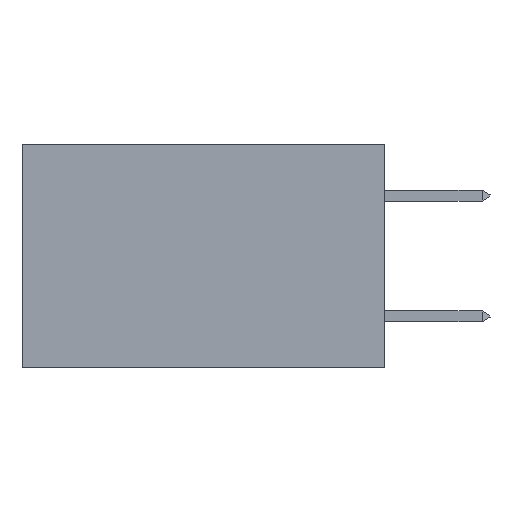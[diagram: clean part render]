
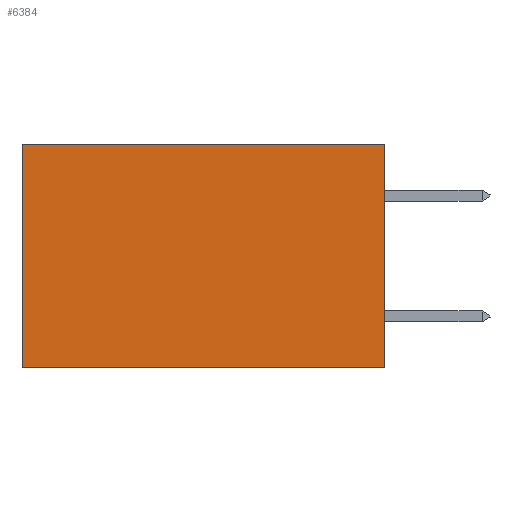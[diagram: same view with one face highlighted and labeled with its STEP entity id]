
A CAD part, left-side view. The second image highlights one B-rep face of the part: STEP entity #6384.
In plain terms, the highlighted planar face has unit normal (-1, 0, 0).
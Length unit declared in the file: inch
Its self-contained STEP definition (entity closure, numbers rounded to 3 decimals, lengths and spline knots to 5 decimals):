
#473 = FACE_OUTER_BOUND ( 'NONE', #5289, .T. ) ;
#729 = VERTEX_POINT ( 'NONE', #10830 ) ;
#1812 = VERTEX_POINT ( 'NONE', #20173 ) ;
#3872 = EDGE_CURVE ( 'NONE', #16620, #5416, #7547, .T. ) ;
#3997 = CARTESIAN_POINT ( 'NONE',  ( 0.2875, 0., 0. ) ) ;
#5289 = EDGE_LOOP ( 'NONE', ( #8280, #13663, #7958, #17122 ) ) ;
#5416 = VERTEX_POINT ( 'NONE', #18683 ) ;
#5691 = LINE ( 'NONE', #11656, #10701 ) ;
#6033 = EDGE_CURVE ( 'NONE', #729, #1812, #9158, .T. ) ;
#6384 = ADVANCED_FACE ( 'NONE', ( #473 ), #18422, .F. ) ;
#6639 = DIRECTION ( 'NONE',  ( 0., 1., 0. ) ) ;
#7234 = AXIS2_PLACEMENT_3D ( 'NONE', #13778, #17371, #12441 ) ;
#7306 = VECTOR ( 'NONE', #18017, 39.37008 ) ;
#7547 = LINE ( 'NONE', #3997, #19393 ) ;
#7958 = ORIENTED_EDGE ( 'NONE', *, *, #3872, .F. ) ;
#8280 = ORIENTED_EDGE ( 'NONE', *, *, #6033, .T. ) ;
#8847 = DIRECTION ( 'NONE',  ( 0., 0., -1. ) ) ;
#9158 = LINE ( 'NONE', #9620, #7306 ) ;
#9620 = CARTESIAN_POINT ( 'NONE',  ( 0.2875, 0.6, 0. ) ) ;
#10701 = VECTOR ( 'NONE', #6639, 39.37008 ) ;
#10830 = CARTESIAN_POINT ( 'NONE',  ( 0.2875, 0.6, 0. ) ) ;
#11576 = EDGE_CURVE ( 'NONE', #5416, #1812, #5691, .T. ) ;
#11656 = CARTESIAN_POINT ( 'NONE',  ( 0.2875, 0., -0.37 ) ) ;
#11910 = VECTOR ( 'NONE', #21262, 39.37008 ) ;
#12441 = DIRECTION ( 'NONE',  ( 0., 0., -1. ) ) ;
#13663 = ORIENTED_EDGE ( 'NONE', *, *, #11576, .F. ) ;
#13744 = LINE ( 'NONE', #16192, #11910 ) ;
#13778 = CARTESIAN_POINT ( 'NONE',  ( 0.2875, 0., 0. ) ) ;
#16192 = CARTESIAN_POINT ( 'NONE',  ( 0.2875, 0., 0. ) ) ;
#16620 = VERTEX_POINT ( 'NONE', #16672 ) ;
#16672 = CARTESIAN_POINT ( 'NONE',  ( 0.2875, 0., 0. ) ) ;
#17122 = ORIENTED_EDGE ( 'NONE', *, *, #20571, .T. ) ;
#17371 = DIRECTION ( 'NONE',  ( 1., 0., 0. ) ) ;
#18017 = DIRECTION ( 'NONE',  ( 0., 0., -1. ) ) ;
#18422 = PLANE ( 'NONE',  #7234 ) ;
#18683 = CARTESIAN_POINT ( 'NONE',  ( 0.2875, 0., -0.37 ) ) ;
#19393 = VECTOR ( 'NONE', #8847, 39.37008 ) ;
#20173 = CARTESIAN_POINT ( 'NONE',  ( 0.2875, 0.6, -0.37 ) ) ;
#20571 = EDGE_CURVE ( 'NONE', #16620, #729, #13744, .T. ) ;
#21262 = DIRECTION ( 'NONE',  ( 0., 1., 0. ) ) ;
